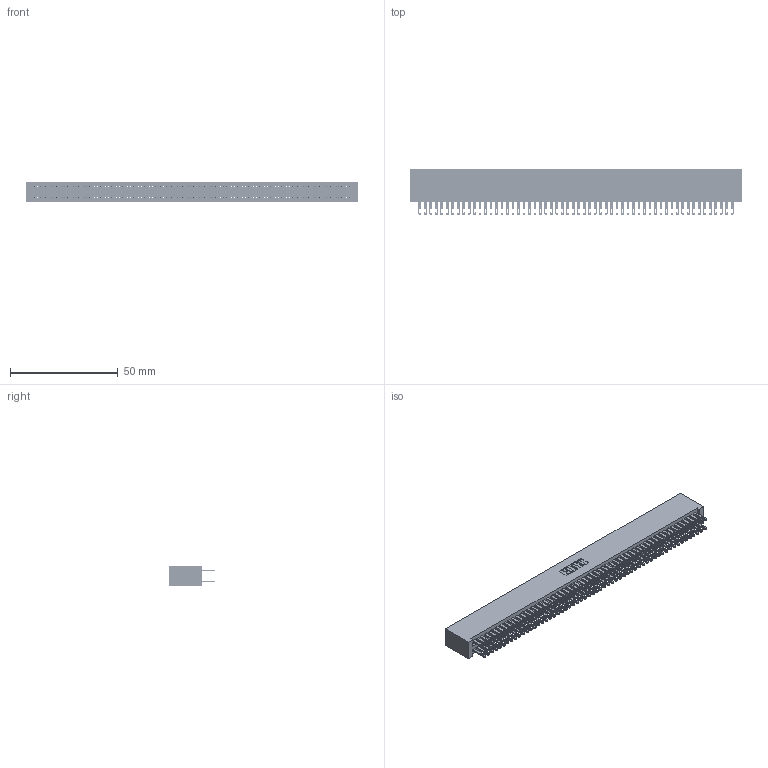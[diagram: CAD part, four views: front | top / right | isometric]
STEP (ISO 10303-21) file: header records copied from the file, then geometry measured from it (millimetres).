
FILE_DESCRIPTION (( 'STEP AP203' ), '1' );
FILE_NAME ('345-116-500-201.STEP', '2019-11-05T13:29:27', ( '' ), ( '' ), 'SwSTEP 2.0', 'SolidWorks 2016', '' );
FILE_SCHEMA (( 'CONFIG_CONTROL_DESIGN' ));
Length unit declared in the file: inch
Products named in the file (3): 345-292-001_345-293-100; 345-116-500-201; 345 Part_No Mounting Lugs
Assembly tree (117 placements, depth 2):
  345-116-500-201
    345 Part_No Mounting Lugs
    345-292-001_345-293-100  x116
Bounding box: 153.92 x 21.51 x 9.4 mm (x, y, z)
Volume: 16071.2 mm3; surface area: 25552.3 mm2
Topology: 117 solids, 117 shells, 5454 faces, 16673 edges, 11114 vertices
Faces by surface type: plane 3208, cylinder 2246
Entity records: 43007 total; most frequent: CARTESIAN_POINT 7192, ORIENTED_EDGE 7126, DIRECTION 6319, EDGE_CURVE 3563, VECTOR 3203, LINE 3203, VERTEX_POINT 2374, AXIS2_PLACEMENT_3D 1558
